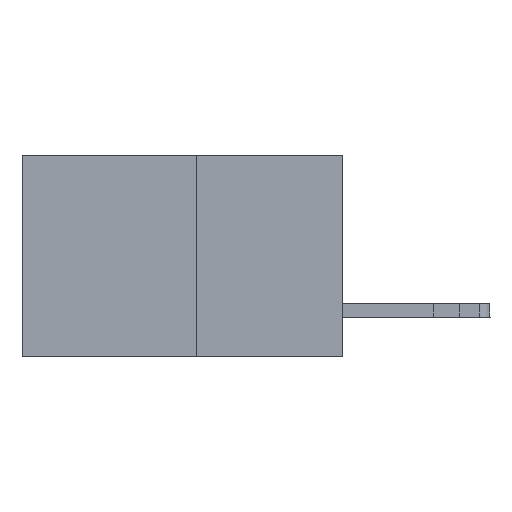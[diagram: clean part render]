
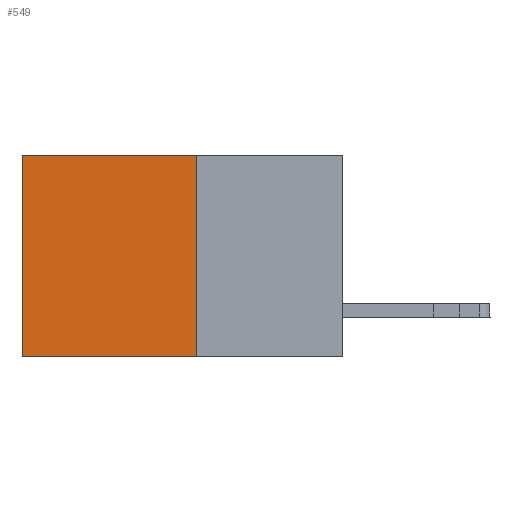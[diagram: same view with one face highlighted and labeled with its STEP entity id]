
A CAD part, left-side view. The second image highlights one B-rep face of the part: STEP entity #549.
In plain terms, the highlighted planar face has unit normal (-1, 0, 0).
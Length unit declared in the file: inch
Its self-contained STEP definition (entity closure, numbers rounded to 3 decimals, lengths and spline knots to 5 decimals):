
#139 = LINE ( 'NONE', #9674, #16353 ) ;
#275 = EDGE_LOOP ( 'NONE', ( #4314, #12825, #15923, #9638 ) ) ;
#500 = EDGE_CURVE ( 'NONE', #8899, #15073, #13263, .T. ) ;
#537 = DIRECTION ( 'NONE',  ( 0., 0., -1. ) ) ;
#549 = ADVANCED_FACE ( 'NONE', ( #2656 ), #16561, .F. ) ;
#752 = VECTOR ( 'NONE', #6026, 39.37008 ) ;
#963 = CARTESIAN_POINT ( 'NONE',  ( 0.277, 0.59, -0.37 ) ) ;
#1742 = DIRECTION ( 'NONE',  ( 1., 0., 0. ) ) ;
#1906 = DIRECTION ( 'NONE',  ( 0., 1., 0. ) ) ;
#2388 = DIRECTION ( 'NONE',  ( 0., 0., -1. ) ) ;
#2623 = VERTEX_POINT ( 'NONE', #2981 ) ;
#2656 = FACE_OUTER_BOUND ( 'NONE', #275, .T. ) ;
#2852 = EDGE_CURVE ( 'NONE', #16513, #15073, #11095, .T. ) ;
#2981 = CARTESIAN_POINT ( 'NONE',  ( 0.277, 0.27, 0. ) ) ;
#4314 = ORIENTED_EDGE ( 'NONE', *, *, #500, .T. ) ;
#5231 = EDGE_CURVE ( 'NONE', #2623, #16513, #8066, .T. ) ;
#6026 = DIRECTION ( 'NONE',  ( 0., 1., 0. ) ) ;
#7335 = CARTESIAN_POINT ( 'NONE',  ( 0.277, 0.27, -0.37 ) ) ;
#7863 = CARTESIAN_POINT ( 'NONE',  ( 0.277, 0.27, -0.37 ) ) ;
#8066 = LINE ( 'NONE', #7863, #11038 ) ;
#8250 = AXIS2_PLACEMENT_3D ( 'NONE', #12000, #1742, #2388 ) ;
#8899 = VERTEX_POINT ( 'NONE', #9235 ) ;
#9071 = CARTESIAN_POINT ( 'NONE',  ( 0.277, 0.27, -0.37 ) ) ;
#9149 = DIRECTION ( 'NONE',  ( 0., 0., -1. ) ) ;
#9235 = CARTESIAN_POINT ( 'NONE',  ( 0.277, 0.59, 0. ) ) ;
#9638 = ORIENTED_EDGE ( 'NONE', *, *, #13061, .T. ) ;
#9674 = CARTESIAN_POINT ( 'NONE',  ( 0.277, 0.27, 0. ) ) ;
#9924 = VECTOR ( 'NONE', #537, 39.37008 ) ;
#11038 = VECTOR ( 'NONE', #9149, 39.37008 ) ;
#11095 = LINE ( 'NONE', #7335, #752 ) ;
#11316 = CARTESIAN_POINT ( 'NONE',  ( 0.277, 0.59, -0.37 ) ) ;
#12000 = CARTESIAN_POINT ( 'NONE',  ( 0.277, 0.27, -0.37 ) ) ;
#12825 = ORIENTED_EDGE ( 'NONE', *, *, #2852, .F. ) ;
#13061 = EDGE_CURVE ( 'NONE', #2623, #8899, #139, .T. ) ;
#13263 = LINE ( 'NONE', #963, #9924 ) ;
#15073 = VERTEX_POINT ( 'NONE', #11316 ) ;
#15923 = ORIENTED_EDGE ( 'NONE', *, *, #5231, .F. ) ;
#16353 = VECTOR ( 'NONE', #1906, 39.37008 ) ;
#16513 = VERTEX_POINT ( 'NONE', #9071 ) ;
#16561 = PLANE ( 'NONE',  #8250 ) ;
